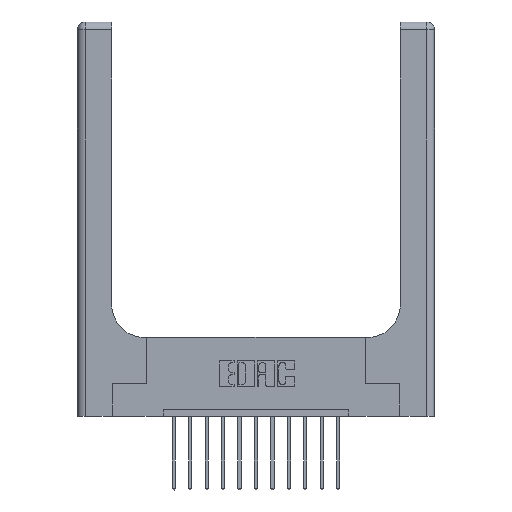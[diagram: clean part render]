
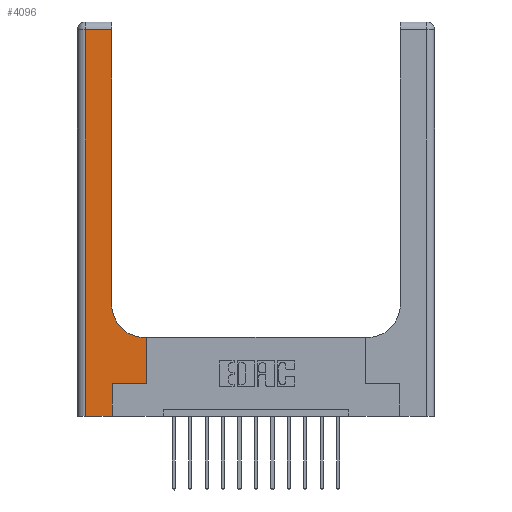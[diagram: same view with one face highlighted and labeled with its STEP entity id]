
A CAD part, top view. The second image highlights one B-rep face of the part: STEP entity #4096.
In plain terms, the highlighted planar face has unit normal (0, 0, 1).
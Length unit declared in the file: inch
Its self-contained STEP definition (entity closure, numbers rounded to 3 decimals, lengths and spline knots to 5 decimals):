
#146 = CARTESIAN_POINT ( 'NONE',  ( 0.265, 0., 0.37 ) ) ;
#458 = DIRECTION ( 'NONE',  ( 0., -1., 0. ) ) ;
#493 = ORIENTED_EDGE ( 'NONE', *, *, #2666, .T. ) ;
#615 = CARTESIAN_POINT ( 'NONE',  ( 0.528, 0.25, 0.37 ) ) ;
#719 = DIRECTION ( 'NONE',  ( 1., 0., 0. ) ) ;
#1124 = LINE ( 'NONE', #10421, #2111 ) ;
#1642 = DIRECTION ( 'NONE',  ( 1., 0., 0. ) ) ;
#2035 = ORIENTED_EDGE ( 'NONE', *, *, #15924, .T. ) ;
#2050 = CARTESIAN_POINT ( 'NONE',  ( 0.26, 2.94, 0.37 ) ) ;
#2111 = VECTOR ( 'NONE', #458, 39.37008 ) ;
#2250 = EDGE_CURVE ( 'NONE', #8779, #8343, #11228, .T. ) ;
#2666 = EDGE_CURVE ( 'NONE', #6444, #4296, #3459, .T. ) ;
#2819 = CARTESIAN_POINT ( 'NONE',  ( 0.26, 0.6, 0.37 ) ) ;
#2948 = CARTESIAN_POINT ( 'NONE',  ( 0.265, 0., 0.37 ) ) ;
#3459 = LINE ( 'NONE', #2819, #5610 ) ;
#3612 = CARTESIAN_POINT ( 'NONE',  ( 0.528, 0.6, 0.37 ) ) ;
#4046 = LINE ( 'NONE', #12320, #12005 ) ;
#4096 = ADVANCED_FACE ( 'NONE', ( #4628 ), #5970, .F. ) ;
#4182 = VERTEX_POINT ( 'NONE', #146 ) ;
#4192 = ORIENTED_EDGE ( 'NONE', *, *, #2250, .T. ) ;
#4208 = DIRECTION ( 'NONE',  ( 0., 1., 0. ) ) ;
#4281 = DIRECTION ( 'NONE',  ( 0., 1., 0. ) ) ;
#4296 = VERTEX_POINT ( 'NONE', #8487 ) ;
#4440 = DIRECTION ( 'NONE',  ( 0., 0., -1. ) ) ;
#4605 = EDGE_LOOP ( 'NONE', ( #8068, #9813, #5915, #5897, #9519, #4192, #5538, #493, #2035 ) ) ;
#4628 = FACE_OUTER_BOUND ( 'NONE', #4605, .T. ) ;
#4681 = CARTESIAN_POINT ( 'NONE',  ( 0.265, 0.25, 0.37 ) ) ;
#4849 = EDGE_CURVE ( 'NONE', #4182, #8779, #15892, .T. ) ;
#5538 = ORIENTED_EDGE ( 'NONE', *, *, #8452, .T. ) ;
#5610 = VECTOR ( 'NONE', #14108, 39.37008 ) ;
#5719 = VERTEX_POINT ( 'NONE', #10585 ) ;
#5897 = ORIENTED_EDGE ( 'NONE', *, *, #7144, .T. ) ;
#5915 = ORIENTED_EDGE ( 'NONE', *, *, #8930, .T. ) ;
#5920 = CARTESIAN_POINT ( 'NONE',  ( 0., 3., 0.37 ) ) ;
#5970 = PLANE ( 'NONE',  #12056 ) ;
#6444 = VERTEX_POINT ( 'NONE', #3612 ) ;
#6873 = CARTESIAN_POINT ( 'NONE',  ( 0.51, 0.85, 0.37 ) ) ;
#6923 = CARTESIAN_POINT ( 'NONE',  ( 0.06, 0., 0.37 ) ) ;
#6986 = LINE ( 'NONE', #13658, #14601 ) ;
#7144 = EDGE_CURVE ( 'NONE', #15958, #4182, #8428, .T. ) ;
#7439 = DIRECTION ( 'NONE',  ( 0., 1., 0. ) ) ;
#7609 = VECTOR ( 'NONE', #4208, 39.37008 ) ;
#7824 = CARTESIAN_POINT ( 'NONE',  ( 0.528, 0.25, 0.37 ) ) ;
#8068 = ORIENTED_EDGE ( 'NONE', *, *, #13151, .T. ) ;
#8197 = CARTESIAN_POINT ( 'NONE',  ( 0.26, 0.85, 0.37 ) ) ;
#8343 = VERTEX_POINT ( 'NONE', #615 ) ;
#8428 = LINE ( 'NONE', #11800, #13118 ) ;
#8452 = EDGE_CURVE ( 'NONE', #8343, #6444, #10709, .T. ) ;
#8487 = CARTESIAN_POINT ( 'NONE',  ( 0.51, 0.6, 0.37 ) ) ;
#8579 = DIRECTION ( 'NONE',  ( -1., 0., 0. ) ) ;
#8698 = AXIS2_PLACEMENT_3D ( 'NONE', #6873, #4440, #11863 ) ;
#8779 = VERTEX_POINT ( 'NONE', #4681 ) ;
#8930 = EDGE_CURVE ( 'NONE', #5719, #15958, #1124, .T. ) ;
#9502 = VECTOR ( 'NONE', #1642, 39.37008 ) ;
#9519 = ORIENTED_EDGE ( 'NONE', *, *, #4849, .T. ) ;
#9813 = ORIENTED_EDGE ( 'NONE', *, *, #14949, .T. ) ;
#10415 = CIRCLE ( 'NONE', #8698, 0.25 ) ;
#10421 = CARTESIAN_POINT ( 'NONE',  ( 0.06, 3., 0.37 ) ) ;
#10585 = CARTESIAN_POINT ( 'NONE',  ( 0.06, 2.94, 0.37 ) ) ;
#10709 = LINE ( 'NONE', #7824, #7609 ) ;
#11228 = LINE ( 'NONE', #15346, #9502 ) ;
#11310 = DIRECTION ( 'NONE',  ( 0., 0., -1. ) ) ;
#11800 = CARTESIAN_POINT ( 'NONE',  ( 0., 0., 0.37 ) ) ;
#11863 = DIRECTION ( 'NONE',  ( 1., 0., 0. ) ) ;
#12005 = VECTOR ( 'NONE', #8579, 39.37008 ) ;
#12056 = AXIS2_PLACEMENT_3D ( 'NONE', #5920, #11310, #15039 ) ;
#12320 = CARTESIAN_POINT ( 'NONE',  ( 0., 2.94, 0.37 ) ) ;
#13025 = VERTEX_POINT ( 'NONE', #2050 ) ;
#13118 = VECTOR ( 'NONE', #719, 39.37008 ) ;
#13151 = EDGE_CURVE ( 'NONE', #13570, #13025, #6986, .T. ) ;
#13570 = VERTEX_POINT ( 'NONE', #8197 ) ;
#13658 = CARTESIAN_POINT ( 'NONE',  ( 0.26, 3., 0.37 ) ) ;
#14108 = DIRECTION ( 'NONE',  ( -1., 0., 0. ) ) ;
#14601 = VECTOR ( 'NONE', #7439, 39.37008 ) ;
#14949 = EDGE_CURVE ( 'NONE', #13025, #5719, #4046, .T. ) ;
#15039 = DIRECTION ( 'NONE',  ( -1., 0., 0. ) ) ;
#15110 = VECTOR ( 'NONE', #4281, 39.37008 ) ;
#15346 = CARTESIAN_POINT ( 'NONE',  ( 0.265, 0.25, 0.37 ) ) ;
#15892 = LINE ( 'NONE', #2948, #15110 ) ;
#15924 = EDGE_CURVE ( 'NONE', #4296, #13570, #10415, .T. ) ;
#15958 = VERTEX_POINT ( 'NONE', #6923 ) ;
